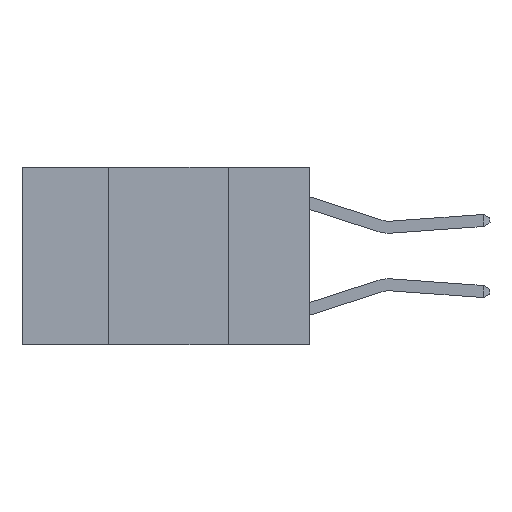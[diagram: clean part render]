
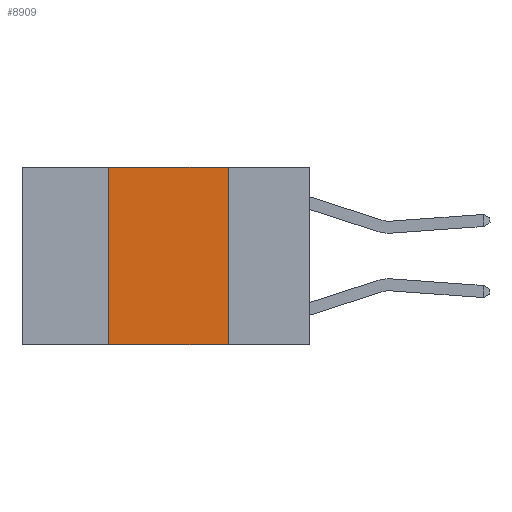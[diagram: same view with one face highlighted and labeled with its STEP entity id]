
A CAD part, left-side view. The second image highlights one B-rep face of the part: STEP entity #8909.
In plain terms, the highlighted planar face has unit normal (-1, 0, 0).
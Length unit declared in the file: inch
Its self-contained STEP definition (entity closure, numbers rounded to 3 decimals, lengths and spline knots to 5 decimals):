
#812 = ORIENTED_EDGE ( 'NONE', *, *, #8093, .F. ) ;
#945 = CARTESIAN_POINT ( 'NONE',  ( 0., 0.42, -0.37 ) ) ;
#1583 = CARTESIAN_POINT ( 'NONE',  ( 0., 0.17, 0. ) ) ;
#1997 = LINE ( 'NONE', #9181, #19208 ) ;
#2220 = VECTOR ( 'NONE', #11668, 39.37008 ) ;
#2266 = CARTESIAN_POINT ( 'NONE',  ( 0., 0.6, -0.37 ) ) ;
#3574 = PLANE ( 'NONE',  #19087 ) ;
#4039 = VECTOR ( 'NONE', #18932, 39.37008 ) ;
#4298 = DIRECTION ( 'NONE',  ( 0., 0., 1. ) ) ;
#4974 = DIRECTION ( 'NONE',  ( 0., 0., -1. ) ) ;
#5252 = DIRECTION ( 'NONE',  ( 0., 0., -1. ) ) ;
#5831 = ORIENTED_EDGE ( 'NONE', *, *, #21564, .F. ) ;
#6405 = VERTEX_POINT ( 'NONE', #945 ) ;
#6874 = ORIENTED_EDGE ( 'NONE', *, *, #11460, .T. ) ;
#8093 = EDGE_CURVE ( 'NONE', #12357, #10473, #15363, .T. ) ;
#8909 = ADVANCED_FACE ( 'NONE', ( #16859 ), #3574, .F. ) ;
#9181 = CARTESIAN_POINT ( 'NONE',  ( 0., 0.42, 0. ) ) ;
#9217 = EDGE_CURVE ( 'NONE', #6405, #14966, #1997, .T. ) ;
#10473 = VERTEX_POINT ( 'NONE', #16589 ) ;
#10950 = VECTOR ( 'NONE', #4974, 39.37008 ) ;
#11460 = EDGE_CURVE ( 'NONE', #6405, #10473, #12897, .T. ) ;
#11668 = DIRECTION ( 'NONE',  ( 0., -1., 0. ) ) ;
#12357 = VERTEX_POINT ( 'NONE', #14795 ) ;
#12897 = LINE ( 'NONE', #2266, #4039 ) ;
#13337 = CARTESIAN_POINT ( 'NONE',  ( 0., 0.6, 0. ) ) ;
#13554 = CARTESIAN_POINT ( 'NONE',  ( 0., 0.6, 0. ) ) ;
#14453 = CARTESIAN_POINT ( 'NONE',  ( 0., 0.42, 0. ) ) ;
#14795 = CARTESIAN_POINT ( 'NONE',  ( 0., 0.17, 0. ) ) ;
#14966 = VERTEX_POINT ( 'NONE', #14453 ) ;
#15032 = LINE ( 'NONE', #13337, #2220 ) ;
#15226 = ORIENTED_EDGE ( 'NONE', *, *, #9217, .F. ) ;
#15250 = DIRECTION ( 'NONE',  ( 1., 0., 0. ) ) ;
#15363 = LINE ( 'NONE', #1583, #10950 ) ;
#16589 = CARTESIAN_POINT ( 'NONE',  ( 0., 0.17, -0.37 ) ) ;
#16859 = FACE_OUTER_BOUND ( 'NONE', #17419, .T. ) ;
#17419 = EDGE_LOOP ( 'NONE', ( #812, #5831, #15226, #6874 ) ) ;
#18932 = DIRECTION ( 'NONE',  ( 0., -1., 0. ) ) ;
#19087 = AXIS2_PLACEMENT_3D ( 'NONE', #13554, #15250, #5252 ) ;
#19208 = VECTOR ( 'NONE', #4298, 39.37008 ) ;
#21564 = EDGE_CURVE ( 'NONE', #14966, #12357, #15032, .T. ) ;
